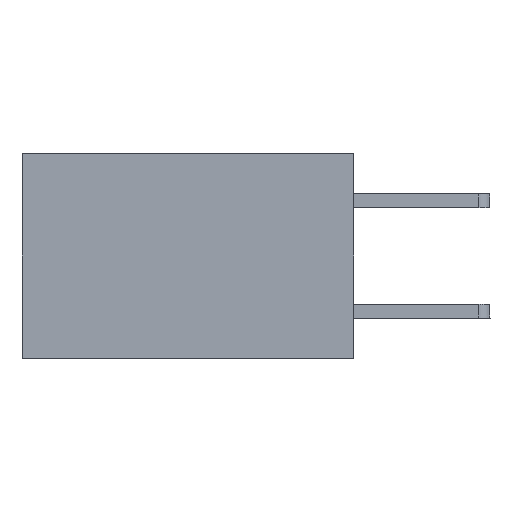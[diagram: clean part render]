
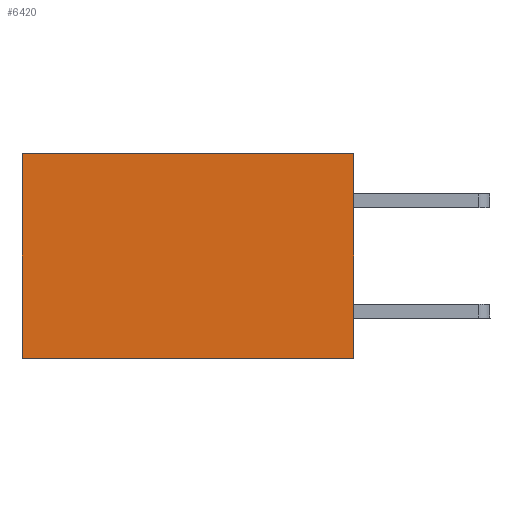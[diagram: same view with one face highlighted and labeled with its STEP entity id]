
A CAD part, left-side view. The second image highlights one B-rep face of the part: STEP entity #6420.
In plain terms, the highlighted planar face has unit normal (-1, 0, 0).
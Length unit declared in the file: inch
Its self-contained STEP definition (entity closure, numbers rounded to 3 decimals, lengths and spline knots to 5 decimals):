
#1 = EDGE_CURVE ( 'NONE', #15821, #15999, #11932, .T. ) ;
#24 = ORIENTED_EDGE ( 'NONE', *, *, #773, .T. ) ;
#599 = DIRECTION ( 'NONE',  ( 0., 0., -1. ) ) ;
#773 = EDGE_CURVE ( 'NONE', #10929, #15821, #17579, .T. ) ;
#912 = LINE ( 'NONE', #17183, #11457 ) ;
#1047 = LINE ( 'NONE', #11610, #14748 ) ;
#2197 = DIRECTION ( 'NONE',  ( 0., 0., -1. ) ) ;
#2306 = EDGE_LOOP ( 'NONE', ( #6748, #7370, #4988, #24 ) ) ;
#4988 = ORIENTED_EDGE ( 'NONE', *, *, #17531, .F. ) ;
#5738 = FACE_OUTER_BOUND ( 'NONE', #2306, .T. ) ;
#5827 = EDGE_CURVE ( 'NONE', #8789, #15999, #912, .T. ) ;
#6420 = ADVANCED_FACE ( 'NONE', ( #5738 ), #7696, .F. ) ;
#6748 = ORIENTED_EDGE ( 'NONE', *, *, #1, .T. ) ;
#6858 = CARTESIAN_POINT ( 'NONE',  ( 0.2875, 0.6, -0.37 ) ) ;
#7370 = ORIENTED_EDGE ( 'NONE', *, *, #5827, .F. ) ;
#7696 = PLANE ( 'NONE',  #11645 ) ;
#7872 = CARTESIAN_POINT ( 'NONE',  ( 0.2875, 0.6, 0. ) ) ;
#8372 = VECTOR ( 'NONE', #13654, 39.37008 ) ;
#8789 = VERTEX_POINT ( 'NONE', #14830 ) ;
#10001 = VECTOR ( 'NONE', #13712, 39.37008 ) ;
#10382 = DIRECTION ( 'NONE',  ( 1., 0., 0. ) ) ;
#10929 = VERTEX_POINT ( 'NONE', #16659 ) ;
#11457 = VECTOR ( 'NONE', #15958, 39.37008 ) ;
#11610 = CARTESIAN_POINT ( 'NONE',  ( 0.2875, 0., 0. ) ) ;
#11645 = AXIS2_PLACEMENT_3D ( 'NONE', #17050, #10382, #2197 ) ;
#11932 = LINE ( 'NONE', #13733, #8372 ) ;
#13654 = DIRECTION ( 'NONE',  ( 0., 0., -1. ) ) ;
#13712 = DIRECTION ( 'NONE',  ( 0., 1., 0. ) ) ;
#13733 = CARTESIAN_POINT ( 'NONE',  ( 0.2875, 0.6, 0. ) ) ;
#13774 = CARTESIAN_POINT ( 'NONE',  ( 0.2875, 0., 0. ) ) ;
#14748 = VECTOR ( 'NONE', #599, 39.37008 ) ;
#14830 = CARTESIAN_POINT ( 'NONE',  ( 0.2875, 0., -0.37 ) ) ;
#15821 = VERTEX_POINT ( 'NONE', #7872 ) ;
#15958 = DIRECTION ( 'NONE',  ( 0., 1., 0. ) ) ;
#15999 = VERTEX_POINT ( 'NONE', #6858 ) ;
#16659 = CARTESIAN_POINT ( 'NONE',  ( 0.2875, 0., 0. ) ) ;
#17050 = CARTESIAN_POINT ( 'NONE',  ( 0.2875, 0., 0. ) ) ;
#17183 = CARTESIAN_POINT ( 'NONE',  ( 0.2875, 0., -0.37 ) ) ;
#17531 = EDGE_CURVE ( 'NONE', #10929, #8789, #1047, .T. ) ;
#17579 = LINE ( 'NONE', #13774, #10001 ) ;
